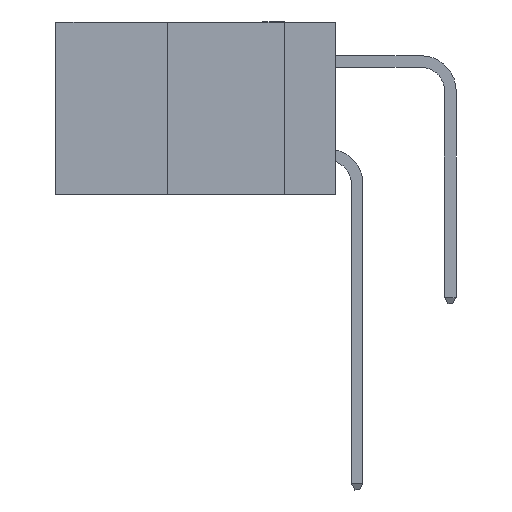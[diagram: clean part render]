
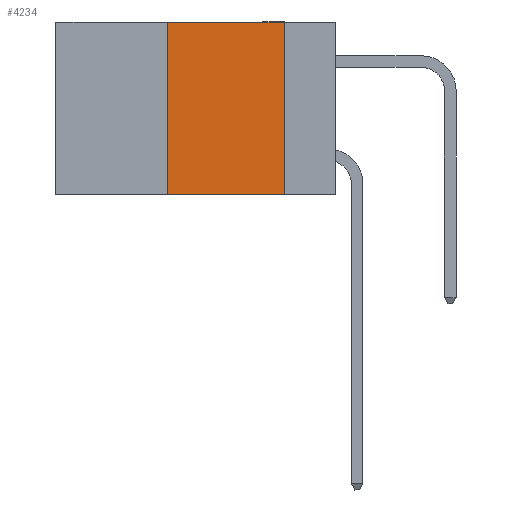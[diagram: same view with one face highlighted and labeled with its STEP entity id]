
A CAD part, left-side view. The second image highlights one B-rep face of the part: STEP entity #4234.
In plain terms, the highlighted planar face has unit normal (-1, 0, 0).
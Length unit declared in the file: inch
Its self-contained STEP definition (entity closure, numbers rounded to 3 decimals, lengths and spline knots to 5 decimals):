
#474 = VERTEX_POINT ( 'NONE', #2747 ) ;
#733 = CARTESIAN_POINT ( 'NONE',  ( 0., 0.36, 0. ) ) ;
#1052 = ORIENTED_EDGE ( 'NONE', *, *, #8115, .T. ) ;
#1121 = DIRECTION ( 'NONE',  ( 0., 0., -1. ) ) ;
#1598 = CARTESIAN_POINT ( 'NONE',  ( 0., 0.11, -0.37 ) ) ;
#2747 = CARTESIAN_POINT ( 'NONE',  ( 0., 0.11, 0. ) ) ;
#3651 = VERTEX_POINT ( 'NONE', #1598 ) ;
#3891 = EDGE_CURVE ( 'NONE', #474, #3651, #15979, .T. ) ;
#4023 = CARTESIAN_POINT ( 'NONE',  ( 0., 0.36, 0. ) ) ;
#4234 = ADVANCED_FACE ( 'NONE', ( #14478 ), #15401, .F. ) ;
#4810 = LINE ( 'NONE', #15702, #15076 ) ;
#4912 = EDGE_CURVE ( 'NONE', #12296, #474, #4810, .T. ) ;
#5444 = EDGE_LOOP ( 'NONE', ( #15618, #11415, #16625, #1052 ) ) ;
#6043 = VECTOR ( 'NONE', #18216, 39.37008 ) ;
#6226 = LINE ( 'NONE', #733, #16825 ) ;
#8115 = EDGE_CURVE ( 'NONE', #14470, #3651, #13448, .T. ) ;
#8656 = VECTOR ( 'NONE', #1121, 39.37008 ) ;
#8762 = EDGE_CURVE ( 'NONE', #14470, #12296, #6226, .T. ) ;
#11129 = DIRECTION ( 'NONE',  ( 1., 0., 0. ) ) ;
#11415 = ORIENTED_EDGE ( 'NONE', *, *, #4912, .F. ) ;
#11787 = AXIS2_PLACEMENT_3D ( 'NONE', #16674, #11129, #12570 ) ;
#12296 = VERTEX_POINT ( 'NONE', #4023 ) ;
#12570 = DIRECTION ( 'NONE',  ( 0., 0., -1. ) ) ;
#13448 = LINE ( 'NONE', #16828, #6043 ) ;
#14220 = DIRECTION ( 'NONE',  ( 0., -1., 0. ) ) ;
#14470 = VERTEX_POINT ( 'NONE', #15901 ) ;
#14478 = FACE_OUTER_BOUND ( 'NONE', #5444, .T. ) ;
#15076 = VECTOR ( 'NONE', #14220, 39.37008 ) ;
#15102 = DIRECTION ( 'NONE',  ( 0., 0., 1. ) ) ;
#15401 = PLANE ( 'NONE',  #11787 ) ;
#15618 = ORIENTED_EDGE ( 'NONE', *, *, #3891, .F. ) ;
#15702 = CARTESIAN_POINT ( 'NONE',  ( 0., 0.6, 0. ) ) ;
#15901 = CARTESIAN_POINT ( 'NONE',  ( 0., 0.36, -0.37 ) ) ;
#15979 = LINE ( 'NONE', #18055, #8656 ) ;
#16625 = ORIENTED_EDGE ( 'NONE', *, *, #8762, .F. ) ;
#16674 = CARTESIAN_POINT ( 'NONE',  ( 0., 0.6, 0. ) ) ;
#16825 = VECTOR ( 'NONE', #15102, 39.37008 ) ;
#16828 = CARTESIAN_POINT ( 'NONE',  ( 0., 0.6, -0.37 ) ) ;
#18055 = CARTESIAN_POINT ( 'NONE',  ( 0., 0.11, 0. ) ) ;
#18216 = DIRECTION ( 'NONE',  ( 0., -1., 0. ) ) ;
